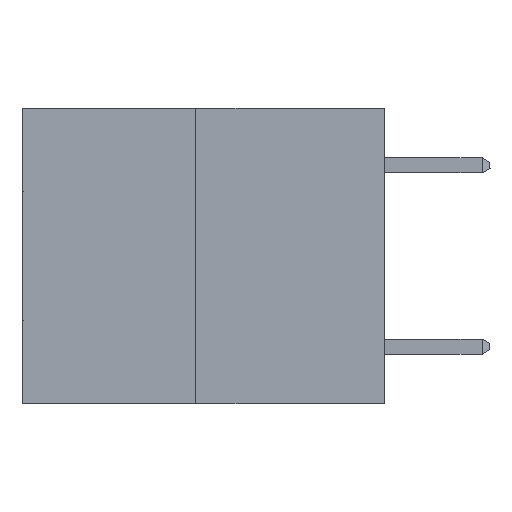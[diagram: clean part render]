
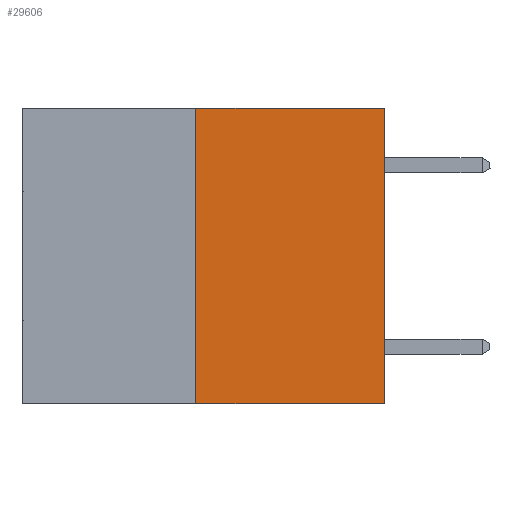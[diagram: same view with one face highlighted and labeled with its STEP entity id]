
A CAD part, left-side view. The second image highlights one B-rep face of the part: STEP entity #29606.
In plain terms, the highlighted planar face has unit normal (-1, 0, 0).
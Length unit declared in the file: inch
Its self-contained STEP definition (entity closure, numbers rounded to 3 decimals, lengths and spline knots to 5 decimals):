
#250 = VECTOR ( 'NONE', #8100, 39.37008 ) ;
#3747 = DIRECTION ( 'NONE',  ( 0., -1., 0. ) ) ;
#3845 = LINE ( 'NONE', #18620, #13412 ) ;
#6006 = VERTEX_POINT ( 'NONE', #14365 ) ;
#6505 = CARTESIAN_POINT ( 'NONE',  ( 0., 0.312, -0.49 ) ) ;
#7122 = LINE ( 'NONE', #8420, #250 ) ;
#7162 = ORIENTED_EDGE ( 'NONE', *, *, #22168, .F. ) ;
#8100 = DIRECTION ( 'NONE',  ( 0., -1., 0. ) ) ;
#8420 = CARTESIAN_POINT ( 'NONE',  ( 0., 0.6, -0.49 ) ) ;
#9094 = ORIENTED_EDGE ( 'NONE', *, *, #21635, .T. ) ;
#11585 = EDGE_LOOP ( 'NONE', ( #7162, #9094, #14712, #18814 ) ) ;
#11622 = VERTEX_POINT ( 'NONE', #19483 ) ;
#11762 = DIRECTION ( 'NONE',  ( 0., 0., -1. ) ) ;
#12009 = EDGE_CURVE ( 'NONE', #11622, #6006, #30868, .T. ) ;
#13412 = VECTOR ( 'NONE', #3747, 39.37008 ) ;
#14128 = DIRECTION ( 'NONE',  ( 1., 0., 0. ) ) ;
#14365 = CARTESIAN_POINT ( 'NONE',  ( 0., 0., 0. ) ) ;
#14712 = ORIENTED_EDGE ( 'NONE', *, *, #12009, .T. ) ;
#15037 = VECTOR ( 'NONE', #28524, 39.37008 ) ;
#16403 = CARTESIAN_POINT ( 'NONE',  ( 0., 0.312, 0. ) ) ;
#16832 = PLANE ( 'NONE',  #19716 ) ;
#18620 = CARTESIAN_POINT ( 'NONE',  ( 0., 0.6, 0. ) ) ;
#18814 = ORIENTED_EDGE ( 'NONE', *, *, #25418, .F. ) ;
#19343 = LINE ( 'NONE', #27614, #28644 ) ;
#19483 = CARTESIAN_POINT ( 'NONE',  ( 0., 0., -0.49 ) ) ;
#19716 = AXIS2_PLACEMENT_3D ( 'NONE', #28922, #14128, #11762 ) ;
#21635 = EDGE_CURVE ( 'NONE', #28181, #11622, #7122, .T. ) ;
#21930 = VERTEX_POINT ( 'NONE', #16403 ) ;
#22168 = EDGE_CURVE ( 'NONE', #28181, #21930, #19343, .T. ) ;
#25418 = EDGE_CURVE ( 'NONE', #21930, #6006, #3845, .T. ) ;
#27495 = FACE_OUTER_BOUND ( 'NONE', #11585, .T. ) ;
#27505 = DIRECTION ( 'NONE',  ( 0., 0., 1. ) ) ;
#27614 = CARTESIAN_POINT ( 'NONE',  ( 0., 0.312, -0.49 ) ) ;
#28181 = VERTEX_POINT ( 'NONE', #6505 ) ;
#28424 = CARTESIAN_POINT ( 'NONE',  ( 0., 0., 0. ) ) ;
#28524 = DIRECTION ( 'NONE',  ( 0., 0., 1. ) ) ;
#28644 = VECTOR ( 'NONE', #27505, 39.37008 ) ;
#28922 = CARTESIAN_POINT ( 'NONE',  ( 0., 0.6, 0. ) ) ;
#29606 = ADVANCED_FACE ( 'NONE', ( #27495 ), #16832, .F. ) ;
#30868 = LINE ( 'NONE', #28424, #15037 ) ;
